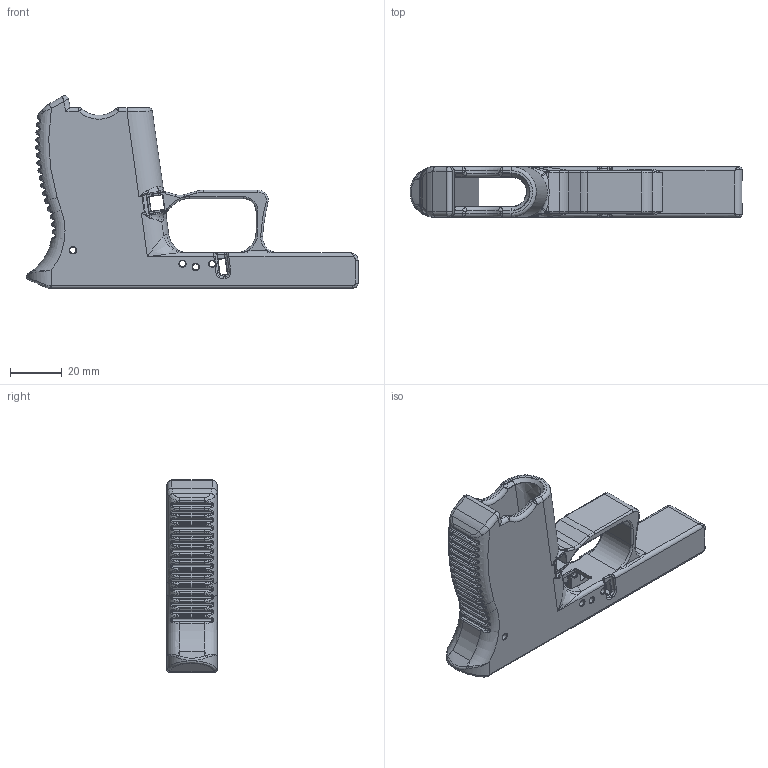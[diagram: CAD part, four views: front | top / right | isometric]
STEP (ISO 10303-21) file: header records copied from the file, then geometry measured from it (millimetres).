
FILE_DESCRIPTION(/* description */ (''),/* implementation_level */ '2;1');
FILE_NAME(/* name */ 'd623bc15-95c4-42d3-85ab-2e918f39d853.stp',/* time_stamp */ '2019-06-02T12:58:02-04:00',/* author */ ('suzuki450ltr'),/* organization */ (''),/* preprocessor_version */ 'ST-DEVELOPER v18',/* originating_system */ 'Autodesk Translation Framework v8.2.0.1029',/* authorisation */ '');
FILE_SCHEMA (('AUTOMOTIVE_DESIGN { 1 0 10303 214 3 1 1 }'));
Products named in the file (1): DB380 Fix
Bounding box: 128.65 x 19.5 x 74.6 mm (x, y, z)
Volume: 45906.2 mm3; surface area: 24918.9 mm2
Topology: 1 solids, 1 shells, 1234 faces, 2969 edges, 1632 vertices
Faces by surface type: bspline 470, cylinder 414, plane 162, torus 138, sphere 29, cone 21
Full cylindrical faces by diameter (mm): 2 x1, 2.35 x8
Entity records: 46440 total; most frequent: CARTESIAN_POINT 20449, ORIENTED_EDGE 5766, DIRECTION 4958, EDGE_CURVE 2883, AXIS2_PLACEMENT_3D 2067, VERTEX_POINT 1632, EDGE_LOOP 1245, FACE_OUTER_BOUND 1234
